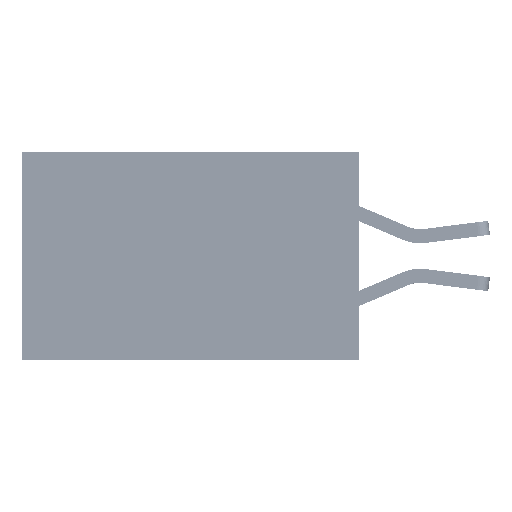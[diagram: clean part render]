
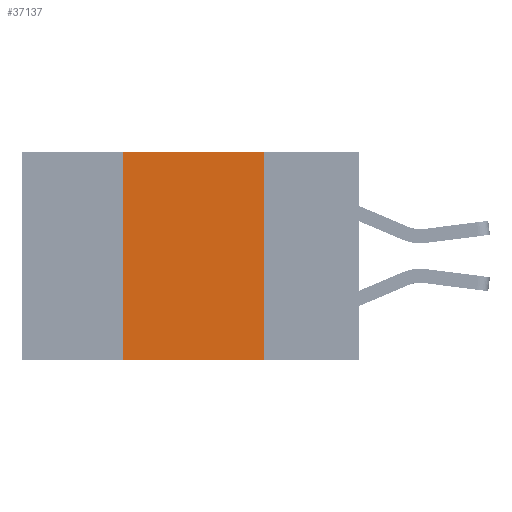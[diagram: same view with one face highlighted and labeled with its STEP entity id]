
A CAD part, left-side view. The second image highlights one B-rep face of the part: STEP entity #37137.
In plain terms, the highlighted planar face has unit normal (-1, 0, 0).
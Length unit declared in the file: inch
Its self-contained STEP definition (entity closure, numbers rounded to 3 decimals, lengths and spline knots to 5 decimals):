
#299 = ORIENTED_EDGE ( 'NONE', *, *, #19888, .T. ) ;
#432 = VECTOR ( 'NONE', #31169, 39.37008 ) ;
#2785 = CARTESIAN_POINT ( 'NONE',  ( 0., 0.6, 0. ) ) ;
#5839 = CARTESIAN_POINT ( 'NONE',  ( 0., 0.17, 0. ) ) ;
#7934 = DIRECTION ( 'NONE',  ( 0., 0., 1. ) ) ;
#9055 = VERTEX_POINT ( 'NONE', #34916 ) ;
#12822 = CARTESIAN_POINT ( 'NONE',  ( 0., 0.6, 0. ) ) ;
#13265 = ORIENTED_EDGE ( 'NONE', *, *, #22215, .F. ) ;
#16025 = FACE_OUTER_BOUND ( 'NONE', #33787, .T. ) ;
#16624 = EDGE_CURVE ( 'NONE', #9055, #39169, #21857, .T. ) ;
#17029 = LINE ( 'NONE', #12822, #26700 ) ;
#17159 = DIRECTION ( 'NONE',  ( 0., -1., 0. ) ) ;
#17476 = PLANE ( 'NONE',  #19480 ) ;
#19239 = LINE ( 'NONE', #46527, #30651 ) ;
#19480 = AXIS2_PLACEMENT_3D ( 'NONE', #2785, #42863, #20994 ) ;
#19785 = EDGE_CURVE ( 'NONE', #33330, #23366, #23841, .T. ) ;
#19888 = EDGE_CURVE ( 'NONE', #9055, #23366, #19239, .T. ) ;
#20994 = DIRECTION ( 'NONE',  ( 0., 0., -1. ) ) ;
#21857 = LINE ( 'NONE', #28262, #36514 ) ;
#22215 = EDGE_CURVE ( 'NONE', #39169, #33330, #17029, .T. ) ;
#23366 = VERTEX_POINT ( 'NONE', #43452 ) ;
#23841 = LINE ( 'NONE', #5839, #432 ) ;
#23879 = ORIENTED_EDGE ( 'NONE', *, *, #19785, .F. ) ;
#25226 = CARTESIAN_POINT ( 'NONE',  ( 0., 0.17, 0. ) ) ;
#26700 = VECTOR ( 'NONE', #28101, 39.37008 ) ;
#28101 = DIRECTION ( 'NONE',  ( 0., -1., 0. ) ) ;
#28262 = CARTESIAN_POINT ( 'NONE',  ( 0., 0.42, 0. ) ) ;
#29670 = CARTESIAN_POINT ( 'NONE',  ( 0., 0.42, 0. ) ) ;
#30651 = VECTOR ( 'NONE', #17159, 39.37008 ) ;
#31169 = DIRECTION ( 'NONE',  ( 0., 0., -1. ) ) ;
#33330 = VERTEX_POINT ( 'NONE', #25226 ) ;
#33787 = EDGE_LOOP ( 'NONE', ( #23879, #13265, #40918, #299 ) ) ;
#34916 = CARTESIAN_POINT ( 'NONE',  ( 0., 0.42, -0.37 ) ) ;
#36514 = VECTOR ( 'NONE', #7934, 39.37008 ) ;
#37137 = ADVANCED_FACE ( 'NONE', ( #16025 ), #17476, .F. ) ;
#39169 = VERTEX_POINT ( 'NONE', #29670 ) ;
#40918 = ORIENTED_EDGE ( 'NONE', *, *, #16624, .F. ) ;
#42863 = DIRECTION ( 'NONE',  ( 1., 0., 0. ) ) ;
#43452 = CARTESIAN_POINT ( 'NONE',  ( 0., 0.17, -0.37 ) ) ;
#46527 = CARTESIAN_POINT ( 'NONE',  ( 0., 0.6, -0.37 ) ) ;
